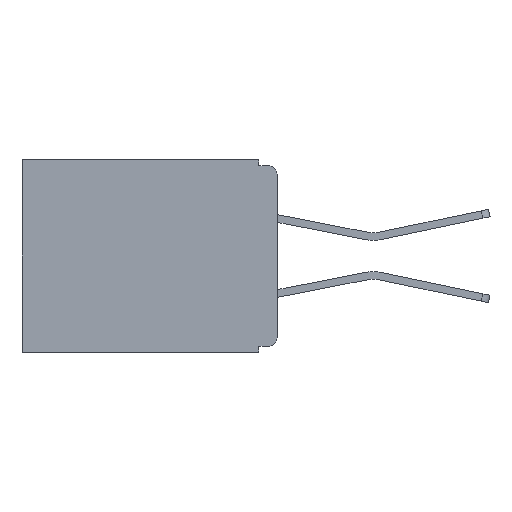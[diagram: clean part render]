
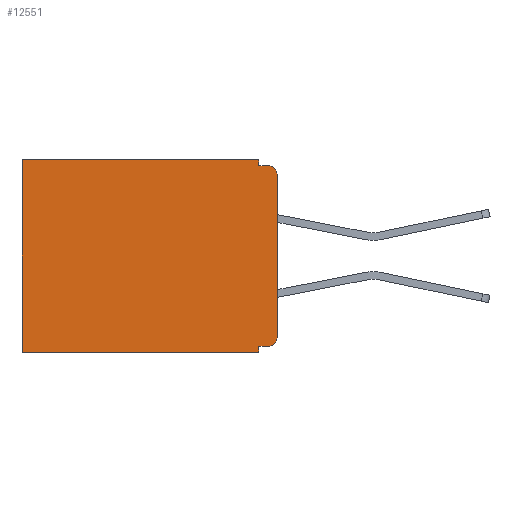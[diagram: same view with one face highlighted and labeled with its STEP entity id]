
A CAD part, left-side view. The second image highlights one B-rep face of the part: STEP entity #12551.
In plain terms, the highlighted planar face has unit normal (-1, 0, 0).
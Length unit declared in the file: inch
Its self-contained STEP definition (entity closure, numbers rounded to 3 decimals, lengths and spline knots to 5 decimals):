
#16 = DIRECTION ( 'NONE',  ( 0., 1., 0. ) ) ;
#290 = ORIENTED_EDGE ( 'NONE', *, *, #19249, .F. ) ;
#769 = CARTESIAN_POINT ( 'NONE',  ( 0.3, 0.437, 0. ) ) ;
#983 = VERTEX_POINT ( 'NONE', #12536 ) ;
#1005 = DIRECTION ( 'NONE',  ( 0., 1., 0. ) ) ;
#2014 = CARTESIAN_POINT ( 'NONE',  ( 0.3, 0., -0.025 ) ) ;
#2141 = AXIS2_PLACEMENT_3D ( 'NONE', #14621, #7949, #23718 ) ;
#2231 = EDGE_CURVE ( 'NONE', #7751, #7468, #16800, .T. ) ;
#2397 = EDGE_CURVE ( 'NONE', #23664, #20570, #7296, .T. ) ;
#2926 = VECTOR ( 'NONE', #10003, 39.37008 ) ;
#3142 = ORIENTED_EDGE ( 'NONE', *, *, #17709, .F. ) ;
#3385 = PLANE ( 'NONE',  #2141 ) ;
#3885 = LINE ( 'NONE', #6728, #9911 ) ;
#4136 = CARTESIAN_POINT ( 'NONE',  ( 0.3, 0., -0.33 ) ) ;
#4807 = VECTOR ( 'NONE', #20395, 39.37008 ) ;
#5463 = EDGE_CURVE ( 'NONE', #983, #18393, #21604, .T. ) ;
#5879 = CARTESIAN_POINT ( 'NONE',  ( 0.3, 0.031, -0.32 ) ) ;
#5905 = VERTEX_POINT ( 'NONE', #13781 ) ;
#5909 = CARTESIAN_POINT ( 'NONE',  ( 0.3, 0.015, -0.01 ) ) ;
#6193 = VECTOR ( 'NONE', #8070, 39.37008 ) ;
#6450 = DIRECTION ( 'NONE',  ( 0., 1., 0. ) ) ;
#6728 = CARTESIAN_POINT ( 'NONE',  ( 0.3, 0., -0.01 ) ) ;
#6916 = LINE ( 'NONE', #10248, #6193 ) ;
#7296 = CIRCLE ( 'NONE', #9374, 0.015 ) ;
#7468 = VERTEX_POINT ( 'NONE', #26080 ) ;
#7593 = CARTESIAN_POINT ( 'NONE',  ( 0.3, 0.031, 0. ) ) ;
#7751 = VERTEX_POINT ( 'NONE', #769 ) ;
#7949 = DIRECTION ( 'NONE',  ( 1., 0., 0. ) ) ;
#8040 = FACE_OUTER_BOUND ( 'NONE', #15927, .T. ) ;
#8070 = DIRECTION ( 'NONE',  ( 0., 0., -1. ) ) ;
#8273 = LINE ( 'NONE', #25739, #2926 ) ;
#8284 = CARTESIAN_POINT ( 'NONE',  ( 0.3, 0., -0.33 ) ) ;
#8672 = VECTOR ( 'NONE', #6450, 39.37008 ) ;
#9371 = VERTEX_POINT ( 'NONE', #16015 ) ;
#9374 = AXIS2_PLACEMENT_3D ( 'NONE', #17588, #26843, #22045 ) ;
#9911 = VECTOR ( 'NONE', #13507, 39.37008 ) ;
#10003 = DIRECTION ( 'NONE',  ( 0., 0., -1. ) ) ;
#10248 = CARTESIAN_POINT ( 'NONE',  ( 0.3, 0.031, -0.33 ) ) ;
#10536 = DIRECTION ( 'NONE',  ( 0., 0., -1. ) ) ;
#11138 = ORIENTED_EDGE ( 'NONE', *, *, #2231, .T. ) ;
#11311 = ORIENTED_EDGE ( 'NONE', *, *, #5463, .F. ) ;
#11447 = ORIENTED_EDGE ( 'NONE', *, *, #28557, .T. ) ;
#11674 = ORIENTED_EDGE ( 'NONE', *, *, #2397, .T. ) ;
#12320 = CARTESIAN_POINT ( 'NONE',  ( 0.3, 0.015, -0.305 ) ) ;
#12328 = CARTESIAN_POINT ( 'NONE',  ( 0.3, 0., -0.32 ) ) ;
#12536 = CARTESIAN_POINT ( 'NONE',  ( 0.3, 0.015, -0.32 ) ) ;
#12551 = ADVANCED_FACE ( 'NONE', ( #8040 ), #3385, .F. ) ;
#12693 = VECTOR ( 'NONE', #16, 39.37008 ) ;
#12764 = VERTEX_POINT ( 'NONE', #15391 ) ;
#13507 = DIRECTION ( 'NONE',  ( 0., -1., 0. ) ) ;
#13626 = CARTESIAN_POINT ( 'NONE',  ( 0.3, 0., 0. ) ) ;
#13781 = CARTESIAN_POINT ( 'NONE',  ( 0.3, 0.031, -0.33 ) ) ;
#13895 = AXIS2_PLACEMENT_3D ( 'NONE', #12320, #27961, #14560 ) ;
#14521 = EDGE_CURVE ( 'NONE', #9371, #20570, #3885, .T. ) ;
#14560 = DIRECTION ( 'NONE',  ( 0., 0., -1. ) ) ;
#14621 = CARTESIAN_POINT ( 'NONE',  ( 0.3, 0., -0.33 ) ) ;
#15391 = CARTESIAN_POINT ( 'NONE',  ( 0.3, 0., -0.305 ) ) ;
#15927 = EDGE_LOOP ( 'NONE', ( #18904, #11674, #19181, #290, #20757, #11138, #21908, #3142, #11311, #11447 ) ) ;
#16015 = CARTESIAN_POINT ( 'NONE',  ( 0.3, 0.031, -0.01 ) ) ;
#16721 = CIRCLE ( 'NONE', #13895, 0.015 ) ;
#16800 = LINE ( 'NONE', #23232, #4807 ) ;
#17588 = CARTESIAN_POINT ( 'NONE',  ( 0.3, 0.015, -0.025 ) ) ;
#17709 = EDGE_CURVE ( 'NONE', #18393, #5905, #6916, .T. ) ;
#17930 = LINE ( 'NONE', #13626, #12693 ) ;
#18393 = VERTEX_POINT ( 'NONE', #5879 ) ;
#18904 = ORIENTED_EDGE ( 'NONE', *, *, #20613, .F. ) ;
#19181 = ORIENTED_EDGE ( 'NONE', *, *, #14521, .F. ) ;
#19249 = EDGE_CURVE ( 'NONE', #23332, #9371, #8273, .T. ) ;
#20395 = DIRECTION ( 'NONE',  ( 0., 0., -1. ) ) ;
#20570 = VERTEX_POINT ( 'NONE', #5909 ) ;
#20613 = EDGE_CURVE ( 'NONE', #23664, #12764, #28520, .T. ) ;
#20757 = ORIENTED_EDGE ( 'NONE', *, *, #26118, .T. ) ;
#20925 = VECTOR ( 'NONE', #1005, 39.37008 ) ;
#21604 = LINE ( 'NONE', #12328, #20925 ) ;
#21908 = ORIENTED_EDGE ( 'NONE', *, *, #28183, .F. ) ;
#21970 = VECTOR ( 'NONE', #10536, 39.37008 ) ;
#22045 = DIRECTION ( 'NONE',  ( 0., 0., -1. ) ) ;
#23232 = CARTESIAN_POINT ( 'NONE',  ( 0.3, 0.437, -0.33 ) ) ;
#23332 = VERTEX_POINT ( 'NONE', #7593 ) ;
#23664 = VERTEX_POINT ( 'NONE', #2014 ) ;
#23718 = DIRECTION ( 'NONE',  ( 0., 0., -1. ) ) ;
#25739 = CARTESIAN_POINT ( 'NONE',  ( 0.3, 0.031, 0. ) ) ;
#25905 = LINE ( 'NONE', #4136, #8672 ) ;
#26080 = CARTESIAN_POINT ( 'NONE',  ( 0.3, 0.437, -0.33 ) ) ;
#26118 = EDGE_CURVE ( 'NONE', #23332, #7751, #17930, .T. ) ;
#26843 = DIRECTION ( 'NONE',  ( -1., 0., 0. ) ) ;
#27961 = DIRECTION ( 'NONE',  ( -1., 0., 0. ) ) ;
#28183 = EDGE_CURVE ( 'NONE', #5905, #7468, #25905, .T. ) ;
#28520 = LINE ( 'NONE', #8284, #21970 ) ;
#28557 = EDGE_CURVE ( 'NONE', #983, #12764, #16721, .T. ) ;
